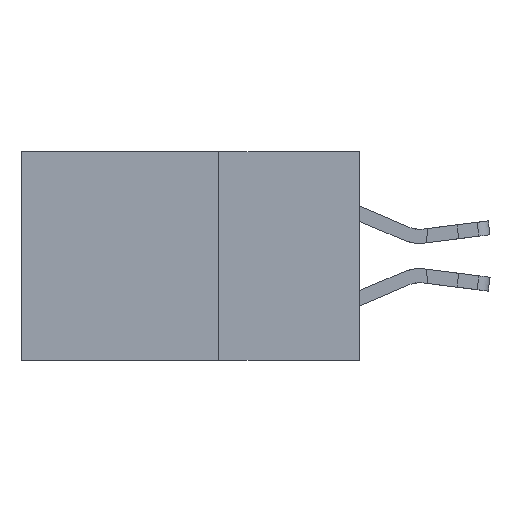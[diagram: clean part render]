
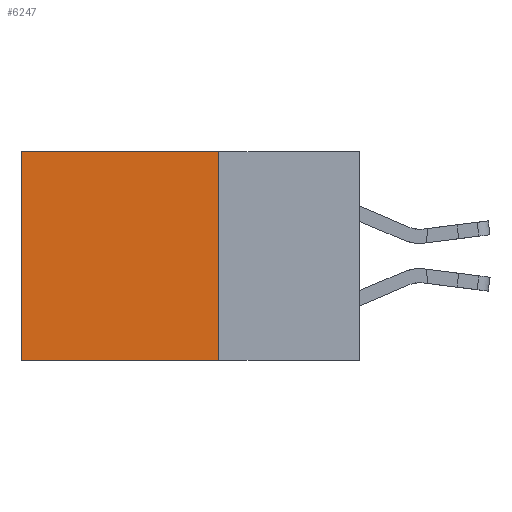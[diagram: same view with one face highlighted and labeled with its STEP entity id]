
A CAD part, left-side view. The second image highlights one B-rep face of the part: STEP entity #6247.
In plain terms, the highlighted planar face has unit normal (-1, 0, 0).
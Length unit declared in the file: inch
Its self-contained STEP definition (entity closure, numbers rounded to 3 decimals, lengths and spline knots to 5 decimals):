
#855 = VERTEX_POINT ( 'NONE', #21584 ) ;
#1014 = LINE ( 'NONE', #24792, #7064 ) ;
#2330 = VERTEX_POINT ( 'NONE', #3462 ) ;
#2737 = LINE ( 'NONE', #11651, #4645 ) ;
#3462 = CARTESIAN_POINT ( 'NONE',  ( 0.2875, 0.6, -0.37 ) ) ;
#4029 = CARTESIAN_POINT ( 'NONE',  ( 0.2875, 0.25, 0. ) ) ;
#4092 = EDGE_CURVE ( 'NONE', #20993, #855, #21269, .T. ) ;
#4611 = EDGE_LOOP ( 'NONE', ( #7593, #25280, #8212, #18739 ) ) ;
#4645 = VECTOR ( 'NONE', #21473, 39.37008 ) ;
#6152 = DIRECTION ( 'NONE',  ( 0., 0., -1. ) ) ;
#6247 = ADVANCED_FACE ( 'NONE', ( #14839 ), #19339, .F. ) ;
#6839 = VECTOR ( 'NONE', #23962, 39.37008 ) ;
#7064 = VECTOR ( 'NONE', #8916, 39.37008 ) ;
#7159 = VECTOR ( 'NONE', #6152, 39.37008 ) ;
#7593 = ORIENTED_EDGE ( 'NONE', *, *, #11647, .T. ) ;
#8212 = ORIENTED_EDGE ( 'NONE', *, *, #4092, .F. ) ;
#8916 = DIRECTION ( 'NONE',  ( 0., 1., 0. ) ) ;
#9467 = CARTESIAN_POINT ( 'NONE',  ( 0.2875, 0.25, 0. ) ) ;
#11372 = VERTEX_POINT ( 'NONE', #19387 ) ;
#11647 = EDGE_CURVE ( 'NONE', #11372, #2330, #24119, .T. ) ;
#11651 = CARTESIAN_POINT ( 'NONE',  ( 0.2875, 0.25, -0.37 ) ) ;
#12295 = CARTESIAN_POINT ( 'NONE',  ( 0.2875, 0.6, 0. ) ) ;
#14214 = DIRECTION ( 'NONE',  ( 1., 0., 0. ) ) ;
#14839 = FACE_OUTER_BOUND ( 'NONE', #4611, .T. ) ;
#15700 = AXIS2_PLACEMENT_3D ( 'NONE', #4029, #14214, #22976 ) ;
#18739 = ORIENTED_EDGE ( 'NONE', *, *, #25762, .T. ) ;
#19339 = PLANE ( 'NONE',  #15700 ) ;
#19387 = CARTESIAN_POINT ( 'NONE',  ( 0.2875, 0.6, 0. ) ) ;
#19777 = CARTESIAN_POINT ( 'NONE',  ( 0.2875, 0.25, 0. ) ) ;
#20993 = VERTEX_POINT ( 'NONE', #9467 ) ;
#21269 = LINE ( 'NONE', #19777, #6839 ) ;
#21473 = DIRECTION ( 'NONE',  ( 0., 1., 0. ) ) ;
#21584 = CARTESIAN_POINT ( 'NONE',  ( 0.2875, 0.25, -0.37 ) ) ;
#22734 = EDGE_CURVE ( 'NONE', #855, #2330, #2737, .T. ) ;
#22976 = DIRECTION ( 'NONE',  ( 0., 0., -1. ) ) ;
#23962 = DIRECTION ( 'NONE',  ( 0., 0., -1. ) ) ;
#24119 = LINE ( 'NONE', #12295, #7159 ) ;
#24792 = CARTESIAN_POINT ( 'NONE',  ( 0.2875, 0.25, 0. ) ) ;
#25280 = ORIENTED_EDGE ( 'NONE', *, *, #22734, .F. ) ;
#25762 = EDGE_CURVE ( 'NONE', #20993, #11372, #1014, .T. ) ;
